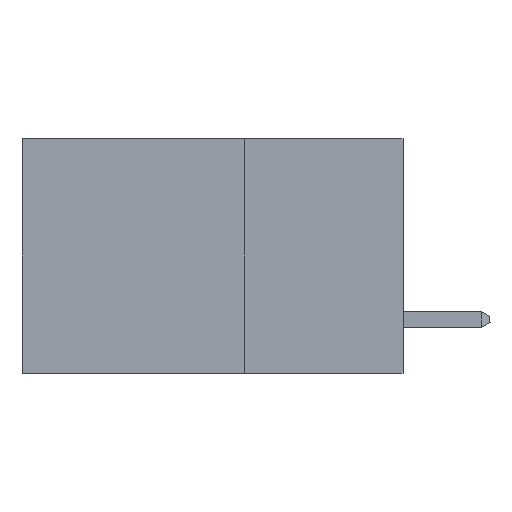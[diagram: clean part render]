
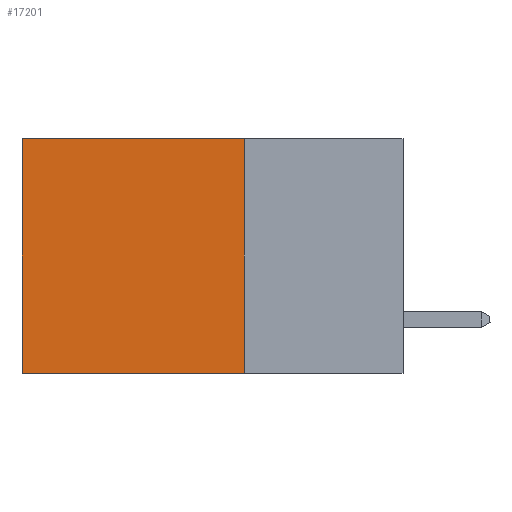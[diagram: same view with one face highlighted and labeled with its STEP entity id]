
A CAD part, left-side view. The second image highlights one B-rep face of the part: STEP entity #17201.
In plain terms, the highlighted planar face has unit normal (-1, 0, 0).
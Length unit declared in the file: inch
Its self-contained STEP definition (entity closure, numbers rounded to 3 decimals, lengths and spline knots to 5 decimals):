
#177 = AXIS2_PLACEMENT_3D ( 'NONE', #19110, #711, #914 ) ;
#711 = DIRECTION ( 'NONE',  ( 1., 0., 0. ) ) ;
#914 = DIRECTION ( 'NONE',  ( 0., 0., -1. ) ) ;
#1115 = LINE ( 'NONE', #10931, #13885 ) ;
#2432 = PLANE ( 'NONE',  #177 ) ;
#3045 = VECTOR ( 'NONE', #14089, 39.37008 ) ;
#3756 = EDGE_CURVE ( 'NONE', #7738, #7905, #9630, .T. ) ;
#4121 = CARTESIAN_POINT ( 'NONE',  ( 0.2875, 0.25, 0. ) ) ;
#4165 = VERTEX_POINT ( 'NONE', #10118 ) ;
#4961 = DIRECTION ( 'NONE',  ( 0., 0., -1. ) ) ;
#5252 = EDGE_CURVE ( 'NONE', #4165, #8576, #17988, .T. ) ;
#6567 = CARTESIAN_POINT ( 'NONE',  ( 0.2875, 0.6, -0.37 ) ) ;
#7738 = VERTEX_POINT ( 'NONE', #16224 ) ;
#7905 = VERTEX_POINT ( 'NONE', #13916 ) ;
#8576 = VERTEX_POINT ( 'NONE', #6567 ) ;
#8844 = ORIENTED_EDGE ( 'NONE', *, *, #15943, .F. ) ;
#8908 = ORIENTED_EDGE ( 'NONE', *, *, #5252, .T. ) ;
#9630 = LINE ( 'NONE', #18683, #9864 ) ;
#9864 = VECTOR ( 'NONE', #4961, 39.37008 ) ;
#10118 = CARTESIAN_POINT ( 'NONE',  ( 0.2875, 0.6, 0. ) ) ;
#10435 = FACE_OUTER_BOUND ( 'NONE', #14036, .T. ) ;
#10898 = ORIENTED_EDGE ( 'NONE', *, *, #3756, .F. ) ;
#10931 = CARTESIAN_POINT ( 'NONE',  ( 0.2875, 0.25, -0.37 ) ) ;
#11001 = EDGE_CURVE ( 'NONE', #7738, #4165, #14320, .T. ) ;
#13885 = VECTOR ( 'NONE', #15584, 39.37008 ) ;
#13916 = CARTESIAN_POINT ( 'NONE',  ( 0.2875, 0.25, -0.37 ) ) ;
#14036 = EDGE_LOOP ( 'NONE', ( #8908, #8844, #10898, #14145 ) ) ;
#14089 = DIRECTION ( 'NONE',  ( 0., 0., -1. ) ) ;
#14145 = ORIENTED_EDGE ( 'NONE', *, *, #11001, .T. ) ;
#14320 = LINE ( 'NONE', #4121, #18163 ) ;
#15584 = DIRECTION ( 'NONE',  ( 0., 1., 0. ) ) ;
#15943 = EDGE_CURVE ( 'NONE', #7905, #8576, #1115, .T. ) ;
#16224 = CARTESIAN_POINT ( 'NONE',  ( 0.2875, 0.25, 0. ) ) ;
#17201 = ADVANCED_FACE ( 'NONE', ( #10435 ), #2432, .F. ) ;
#17988 = LINE ( 'NONE', #18957, #3045 ) ;
#17998 = DIRECTION ( 'NONE',  ( 0., 1., 0. ) ) ;
#18163 = VECTOR ( 'NONE', #17998, 39.37008 ) ;
#18683 = CARTESIAN_POINT ( 'NONE',  ( 0.2875, 0.25, 0. ) ) ;
#18957 = CARTESIAN_POINT ( 'NONE',  ( 0.2875, 0.6, 0. ) ) ;
#19110 = CARTESIAN_POINT ( 'NONE',  ( 0.2875, 0.25, 0. ) ) ;
